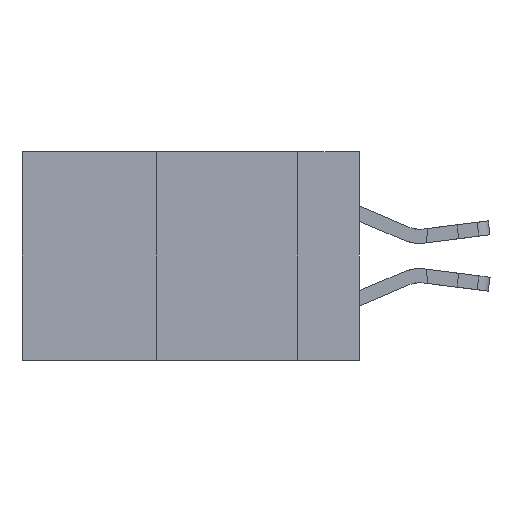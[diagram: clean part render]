
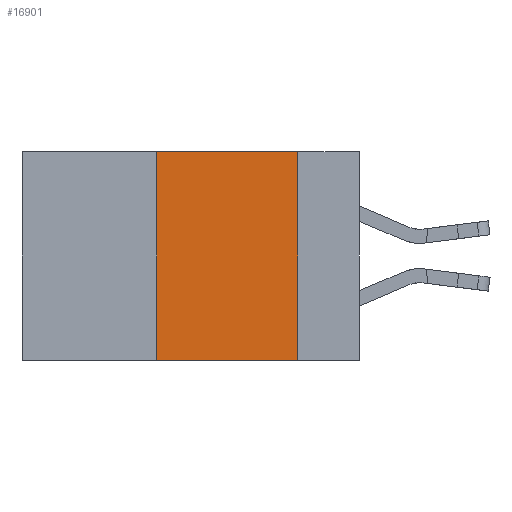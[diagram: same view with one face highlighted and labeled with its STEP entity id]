
A CAD part, left-side view. The second image highlights one B-rep face of the part: STEP entity #16901.
In plain terms, the highlighted planar face has unit normal (-1, 0, 0).
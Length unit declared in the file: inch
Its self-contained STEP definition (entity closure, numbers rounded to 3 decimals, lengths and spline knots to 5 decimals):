
#1354 = VECTOR ( 'NONE', #14673, 39.37008 ) ;
#3011 = CARTESIAN_POINT ( 'NONE',  ( 0., 0.6, -0.37 ) ) ;
#3494 = LINE ( 'NONE', #6582, #1354 ) ;
#3771 = VECTOR ( 'NONE', #15539, 39.37008 ) ;
#3858 = ORIENTED_EDGE ( 'NONE', *, *, #6916, .F. ) ;
#4319 = CARTESIAN_POINT ( 'NONE',  ( 0., 0.11, 0. ) ) ;
#4493 = DIRECTION ( 'NONE',  ( 0., 0., 1. ) ) ;
#5142 = VERTEX_POINT ( 'NONE', #13814 ) ;
#5993 = VERTEX_POINT ( 'NONE', #4319 ) ;
#6582 = CARTESIAN_POINT ( 'NONE',  ( 0., 0.11, 0. ) ) ;
#6916 = EDGE_CURVE ( 'NONE', #5142, #7301, #15159, .T. ) ;
#7168 = LINE ( 'NONE', #3011, #3771 ) ;
#7301 = VERTEX_POINT ( 'NONE', #14119 ) ;
#7646 = LINE ( 'NONE', #11832, #16392 ) ;
#8140 = AXIS2_PLACEMENT_3D ( 'NONE', #15527, #8826, #11389 ) ;
#8282 = FACE_OUTER_BOUND ( 'NONE', #13779, .T. ) ;
#8826 = DIRECTION ( 'NONE',  ( 1., 0., 0. ) ) ;
#9129 = VERTEX_POINT ( 'NONE', #16005 ) ;
#9725 = CARTESIAN_POINT ( 'NONE',  ( 0., 0.36, 0. ) ) ;
#10081 = PLANE ( 'NONE',  #8140 ) ;
#11389 = DIRECTION ( 'NONE',  ( 0., 0., -1. ) ) ;
#11519 = VECTOR ( 'NONE', #4493, 39.37008 ) ;
#11832 = CARTESIAN_POINT ( 'NONE',  ( 0., 0.6, 0. ) ) ;
#13500 = EDGE_CURVE ( 'NONE', #5993, #9129, #3494, .T. ) ;
#13779 = EDGE_LOOP ( 'NONE', ( #13892, #16312, #3858, #14114 ) ) ;
#13814 = CARTESIAN_POINT ( 'NONE',  ( 0., 0.36, -0.37 ) ) ;
#13892 = ORIENTED_EDGE ( 'NONE', *, *, #13500, .F. ) ;
#14114 = ORIENTED_EDGE ( 'NONE', *, *, #17492, .T. ) ;
#14119 = CARTESIAN_POINT ( 'NONE',  ( 0., 0.36, 0. ) ) ;
#14673 = DIRECTION ( 'NONE',  ( 0., 0., -1. ) ) ;
#15159 = LINE ( 'NONE', #9725, #11519 ) ;
#15527 = CARTESIAN_POINT ( 'NONE',  ( 0., 0.6, 0. ) ) ;
#15539 = DIRECTION ( 'NONE',  ( 0., -1., 0. ) ) ;
#16005 = CARTESIAN_POINT ( 'NONE',  ( 0., 0.11, -0.37 ) ) ;
#16231 = DIRECTION ( 'NONE',  ( 0., -1., 0. ) ) ;
#16312 = ORIENTED_EDGE ( 'NONE', *, *, #16415, .F. ) ;
#16392 = VECTOR ( 'NONE', #16231, 39.37008 ) ;
#16415 = EDGE_CURVE ( 'NONE', #7301, #5993, #7646, .T. ) ;
#16901 = ADVANCED_FACE ( 'NONE', ( #8282 ), #10081, .F. ) ;
#17492 = EDGE_CURVE ( 'NONE', #5142, #9129, #7168, .T. ) ;
